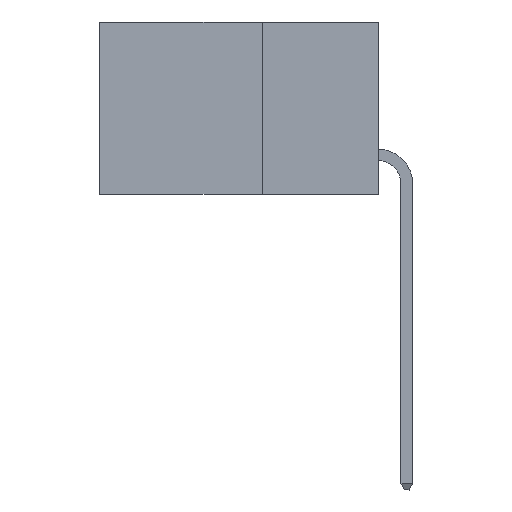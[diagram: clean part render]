
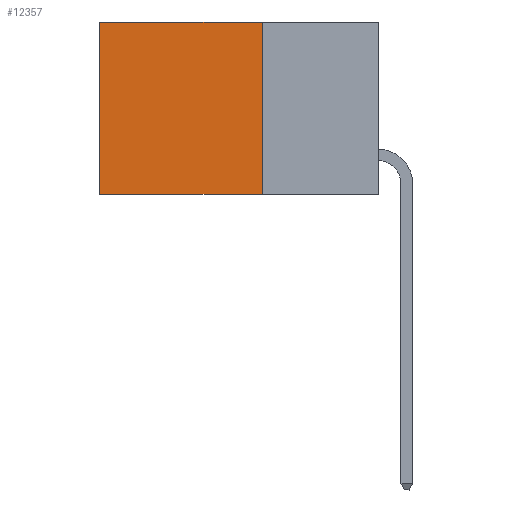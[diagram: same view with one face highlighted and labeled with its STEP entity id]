
A CAD part, left-side view. The second image highlights one B-rep face of the part: STEP entity #12357.
In plain terms, the highlighted planar face has unit normal (-1, 0, 0).
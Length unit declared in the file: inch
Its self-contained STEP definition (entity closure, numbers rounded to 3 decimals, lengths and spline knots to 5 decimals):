
#190 = CARTESIAN_POINT ( 'NONE',  ( 0.2615, 0.25, -0.37 ) ) ;
#676 = CARTESIAN_POINT ( 'NONE',  ( 0.2615, 0.25, -0.37 ) ) ;
#1844 = DIRECTION ( 'NONE',  ( 0., 1., 0. ) ) ;
#1866 = LINE ( 'NONE', #190, #16205 ) ;
#2162 = CARTESIAN_POINT ( 'NONE',  ( 0.2615, 0.25, -0.37 ) ) ;
#4446 = LINE ( 'NONE', #14046, #14696 ) ;
#5756 = VECTOR ( 'NONE', #1844, 39.37008 ) ;
#5885 = ORIENTED_EDGE ( 'NONE', *, *, #16500, .T. ) ;
#7076 = VERTEX_POINT ( 'NONE', #15853 ) ;
#8224 = VERTEX_POINT ( 'NONE', #8314 ) ;
#8314 = CARTESIAN_POINT ( 'NONE',  ( 0.2615, 0.25, 0. ) ) ;
#9275 = EDGE_CURVE ( 'NONE', #20561, #7076, #4446, .T. ) ;
#9428 = CARTESIAN_POINT ( 'NONE',  ( 0.2615, 0.6, 0. ) ) ;
#10157 = ORIENTED_EDGE ( 'NONE', *, *, #13458, .F. ) ;
#10286 = FACE_OUTER_BOUND ( 'NONE', #12002, .T. ) ;
#10637 = ORIENTED_EDGE ( 'NONE', *, *, #9275, .T. ) ;
#12002 = EDGE_LOOP ( 'NONE', ( #10637, #10157, #13310, #5885 ) ) ;
#12293 = PLANE ( 'NONE',  #13494 ) ;
#12357 = ADVANCED_FACE ( 'NONE', ( #10286 ), #12293, .F. ) ;
#12367 = CARTESIAN_POINT ( 'NONE',  ( 0.2615, 0.25, 0. ) ) ;
#13268 = CARTESIAN_POINT ( 'NONE',  ( 0.2615, 0.25, -0.37 ) ) ;
#13310 = ORIENTED_EDGE ( 'NONE', *, *, #17029, .F. ) ;
#13458 = EDGE_CURVE ( 'NONE', #20294, #7076, #16655, .T. ) ;
#13494 = AXIS2_PLACEMENT_3D ( 'NONE', #676, #16746, #18770 ) ;
#14046 = CARTESIAN_POINT ( 'NONE',  ( 0.2615, 0.6, -0.37 ) ) ;
#14696 = VECTOR ( 'NONE', #19047, 39.37008 ) ;
#15853 = CARTESIAN_POINT ( 'NONE',  ( 0.2615, 0.6, -0.37 ) ) ;
#16071 = LINE ( 'NONE', #12367, #17194 ) ;
#16205 = VECTOR ( 'NONE', #19787, 39.37008 ) ;
#16500 = EDGE_CURVE ( 'NONE', #8224, #20561, #16071, .T. ) ;
#16655 = LINE ( 'NONE', #2162, #5756 ) ;
#16746 = DIRECTION ( 'NONE',  ( 1., 0., 0. ) ) ;
#17029 = EDGE_CURVE ( 'NONE', #8224, #20294, #1866, .T. ) ;
#17194 = VECTOR ( 'NONE', #19065, 39.37008 ) ;
#18770 = DIRECTION ( 'NONE',  ( 0., 0., -1. ) ) ;
#19047 = DIRECTION ( 'NONE',  ( 0., 0., -1. ) ) ;
#19065 = DIRECTION ( 'NONE',  ( 0., 1., 0. ) ) ;
#19787 = DIRECTION ( 'NONE',  ( 0., 0., -1. ) ) ;
#20294 = VERTEX_POINT ( 'NONE', #13268 ) ;
#20561 = VERTEX_POINT ( 'NONE', #9428 ) ;
